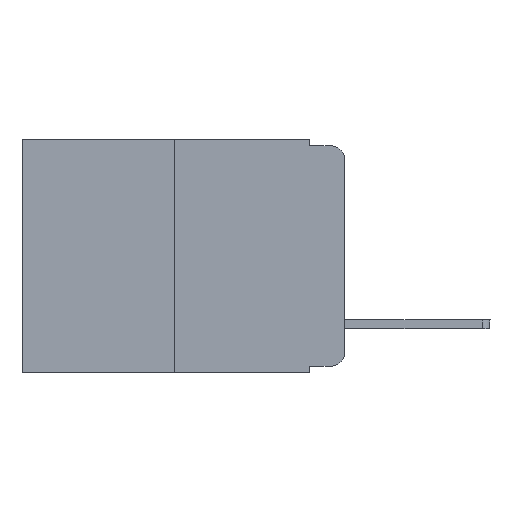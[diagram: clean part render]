
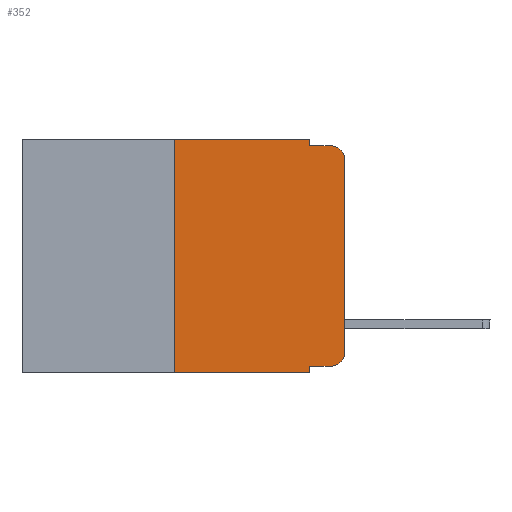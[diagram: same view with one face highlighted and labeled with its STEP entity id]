
A CAD part, left-side view. The second image highlights one B-rep face of the part: STEP entity #352.
In plain terms, the highlighted planar face has unit normal (-1, 0, 0).
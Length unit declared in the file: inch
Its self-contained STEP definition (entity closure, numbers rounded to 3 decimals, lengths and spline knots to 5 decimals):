
#352 = ADVANCED_FACE ( 'NONE', ( #2142 ), #20086, .F. ) ;
#389 = ORIENTED_EDGE ( 'NONE', *, *, #17200, .T. ) ;
#631 = VERTEX_POINT ( 'NONE', #14628 ) ;
#710 = EDGE_CURVE ( 'NONE', #5888, #20856, #13483, .T. ) ;
#789 = LINE ( 'NONE', #1000, #15323 ) ;
#836 = EDGE_CURVE ( 'NONE', #20856, #15020, #12404, .T. ) ;
#950 = DIRECTION ( 'NONE',  ( 0., -1., 0. ) ) ;
#1000 = CARTESIAN_POINT ( 'NONE',  ( 0., 0.051, 0. ) ) ;
#1898 = AXIS2_PLACEMENT_3D ( 'NONE', #13297, #3757, #9897 ) ;
#1918 = CARTESIAN_POINT ( 'NONE',  ( 0., 0.051, 0. ) ) ;
#2142 = FACE_OUTER_BOUND ( 'NONE', #15672, .T. ) ;
#2178 = LINE ( 'NONE', #14805, #15479 ) ;
#2564 = VECTOR ( 'NONE', #7301, 39.37008 ) ;
#2865 = EDGE_CURVE ( 'NONE', #14175, #631, #2178, .T. ) ;
#3695 = LINE ( 'NONE', #16633, #2564 ) ;
#3757 = DIRECTION ( 'NONE',  ( -1., 0., 0. ) ) ;
#3887 = DIRECTION ( 'NONE',  ( 0., 0., 1. ) ) ;
#3957 = VECTOR ( 'NONE', #17047, 39.37008 ) ;
#4005 = DIRECTION ( 'NONE',  ( -1., 0., 0. ) ) ;
#4112 = ORIENTED_EDGE ( 'NONE', *, *, #18804, .T. ) ;
#4711 = VERTEX_POINT ( 'NONE', #17829 ) ;
#4930 = CIRCLE ( 'NONE', #10701, 0.02 ) ;
#5157 = EDGE_CURVE ( 'NONE', #18398, #13252, #18570, .T. ) ;
#5294 = CARTESIAN_POINT ( 'NONE',  ( 0., 0., -0.313 ) ) ;
#5407 = CARTESIAN_POINT ( 'NONE',  ( 0., 0.051, 0. ) ) ;
#5888 = VERTEX_POINT ( 'NONE', #1918 ) ;
#6444 = EDGE_CURVE ( 'NONE', #14175, #7063, #3695, .T. ) ;
#6942 = DIRECTION ( 'NONE',  ( 0., -1., 0. ) ) ;
#7063 = VERTEX_POINT ( 'NONE', #7479 ) ;
#7119 = ORIENTED_EDGE ( 'NONE', *, *, #16641, .F. ) ;
#7301 = DIRECTION ( 'NONE',  ( 0., -1., 0. ) ) ;
#7479 = CARTESIAN_POINT ( 'NONE',  ( 0., 0.051, -0.343 ) ) ;
#8729 = DIRECTION ( 'NONE',  ( 1., 0., 0. ) ) ;
#9897 = DIRECTION ( 'NONE',  ( 0., 0., -1. ) ) ;
#9994 = VECTOR ( 'NONE', #13034, 39.37008 ) ;
#10169 = CARTESIAN_POINT ( 'NONE',  ( 0., 0.051, -0.01 ) ) ;
#10337 = CARTESIAN_POINT ( 'NONE',  ( 0., 0.051, -0.333 ) ) ;
#10701 = AXIS2_PLACEMENT_3D ( 'NONE', #13543, #4005, #20128 ) ;
#10787 = CARTESIAN_POINT ( 'NONE',  ( 0., 0., -0.03 ) ) ;
#10805 = CARTESIAN_POINT ( 'NONE',  ( 0., 0.051, -0.01 ) ) ;
#10840 = LINE ( 'NONE', #19623, #9994 ) ;
#11722 = VECTOR ( 'NONE', #6942, 39.37008 ) ;
#11802 = DIRECTION ( 'NONE',  ( 0., 0., -1. ) ) ;
#11937 = VERTEX_POINT ( 'NONE', #13362 ) ;
#12156 = ORIENTED_EDGE ( 'NONE', *, *, #710, .F. ) ;
#12404 = LINE ( 'NONE', #10805, #18109 ) ;
#13034 = DIRECTION ( 'NONE',  ( 0., -1., 0. ) ) ;
#13252 = VERTEX_POINT ( 'NONE', #10787 ) ;
#13294 = ORIENTED_EDGE ( 'NONE', *, *, #18869, .T. ) ;
#13297 = CARTESIAN_POINT ( 'NONE',  ( 0., 0.02, -0.03 ) ) ;
#13362 = CARTESIAN_POINT ( 'NONE',  ( 0., 0.02, -0.333 ) ) ;
#13483 = LINE ( 'NONE', #5407, #19181 ) ;
#13538 = EDGE_CURVE ( 'NONE', #4711, #7063, #789, .T. ) ;
#13543 = CARTESIAN_POINT ( 'NONE',  ( 0., 0.02, -0.313 ) ) ;
#14175 = VERTEX_POINT ( 'NONE', #19425 ) ;
#14628 = CARTESIAN_POINT ( 'NONE',  ( 0., 0.25, 0. ) ) ;
#14790 = LINE ( 'NONE', #10337, #11722 ) ;
#14805 = CARTESIAN_POINT ( 'NONE',  ( 0., 0.25, 0. ) ) ;
#14848 = DIRECTION ( 'NONE',  ( 0., 0., -1. ) ) ;
#15020 = VERTEX_POINT ( 'NONE', #18181 ) ;
#15084 = AXIS2_PLACEMENT_3D ( 'NONE', #19976, #8729, #11802 ) ;
#15323 = VECTOR ( 'NONE', #20634, 39.37008 ) ;
#15479 = VECTOR ( 'NONE', #3887, 39.37008 ) ;
#15672 = EDGE_LOOP ( 'NONE', ( #16558, #13294, #15971, #12156, #7119, #16508, #17685, #19805, #4112, #389 ) ) ;
#15971 = ORIENTED_EDGE ( 'NONE', *, *, #836, .F. ) ;
#16508 = ORIENTED_EDGE ( 'NONE', *, *, #2865, .F. ) ;
#16558 = ORIENTED_EDGE ( 'NONE', *, *, #5157, .T. ) ;
#16633 = CARTESIAN_POINT ( 'NONE',  ( 0., 0.473, -0.343 ) ) ;
#16641 = EDGE_CURVE ( 'NONE', #631, #5888, #10840, .T. ) ;
#16813 = CIRCLE ( 'NONE', #1898, 0.02 ) ;
#17047 = DIRECTION ( 'NONE',  ( 0., 0., 1. ) ) ;
#17200 = EDGE_CURVE ( 'NONE', #11937, #18398, #4930, .T. ) ;
#17685 = ORIENTED_EDGE ( 'NONE', *, *, #6444, .T. ) ;
#17829 = CARTESIAN_POINT ( 'NONE',  ( 0., 0.051, -0.333 ) ) ;
#18109 = VECTOR ( 'NONE', #950, 39.37008 ) ;
#18181 = CARTESIAN_POINT ( 'NONE',  ( 0., 0.02, -0.01 ) ) ;
#18398 = VERTEX_POINT ( 'NONE', #5294 ) ;
#18570 = LINE ( 'NONE', #20148, #3957 ) ;
#18804 = EDGE_CURVE ( 'NONE', #4711, #11937, #14790, .T. ) ;
#18869 = EDGE_CURVE ( 'NONE', #13252, #15020, #16813, .T. ) ;
#19181 = VECTOR ( 'NONE', #14848, 39.37008 ) ;
#19425 = CARTESIAN_POINT ( 'NONE',  ( 0., 0.25, -0.343 ) ) ;
#19623 = CARTESIAN_POINT ( 'NONE',  ( 0., 0.473, 0. ) ) ;
#19805 = ORIENTED_EDGE ( 'NONE', *, *, #13538, .F. ) ;
#19976 = CARTESIAN_POINT ( 'NONE',  ( 0., 0.473, 0. ) ) ;
#20086 = PLANE ( 'NONE',  #15084 ) ;
#20128 = DIRECTION ( 'NONE',  ( 0., 0., -1. ) ) ;
#20148 = CARTESIAN_POINT ( 'NONE',  ( 0., 0., 0. ) ) ;
#20634 = DIRECTION ( 'NONE',  ( 0., 0., -1. ) ) ;
#20856 = VERTEX_POINT ( 'NONE', #10169 ) ;
